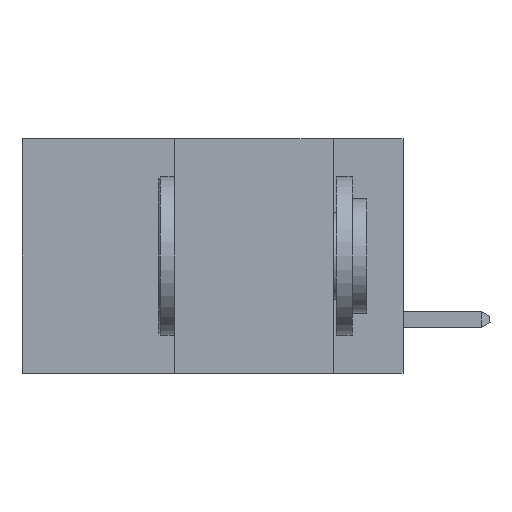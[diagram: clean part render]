
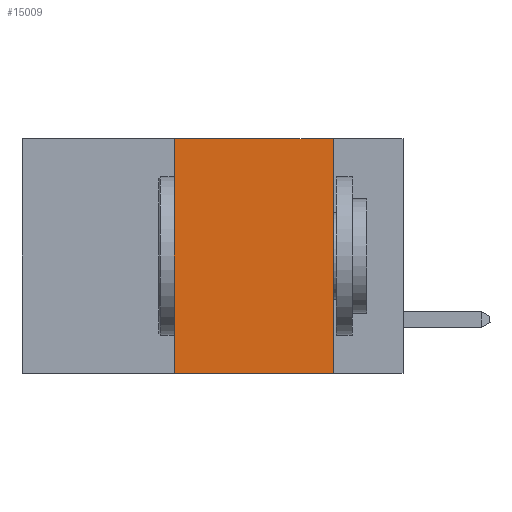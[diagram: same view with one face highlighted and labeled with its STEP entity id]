
A CAD part, left-side view. The second image highlights one B-rep face of the part: STEP entity #15009.
In plain terms, the highlighted planar face has unit normal (-1, 0, 0).
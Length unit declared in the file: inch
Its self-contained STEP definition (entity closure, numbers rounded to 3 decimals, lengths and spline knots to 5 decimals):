
#954 = EDGE_CURVE ( 'NONE', #8883, #10786, #8294, .T. ) ;
#1564 = ORIENTED_EDGE ( 'NONE', *, *, #954, .F. ) ;
#3146 = CARTESIAN_POINT ( 'NONE',  ( 0., 0.11, -0.37 ) ) ;
#3735 = DIRECTION ( 'NONE',  ( 0., -1., 0. ) ) ;
#4073 = VECTOR ( 'NONE', #7218, 39.37008 ) ;
#4391 = CARTESIAN_POINT ( 'NONE',  ( 0., 0.6, 0. ) ) ;
#4557 = ORIENTED_EDGE ( 'NONE', *, *, #16565, .T. ) ;
#4887 = CARTESIAN_POINT ( 'NONE',  ( 0., 0.36, -0.37 ) ) ;
#5022 = EDGE_LOOP ( 'NONE', ( #1564, #17696, #13849, #4557 ) ) ;
#5976 = FACE_OUTER_BOUND ( 'NONE', #5022, .T. ) ;
#6157 = DIRECTION ( 'NONE',  ( 0., 0., 1. ) ) ;
#6359 = VECTOR ( 'NONE', #3735, 39.37008 ) ;
#6648 = DIRECTION ( 'NONE',  ( 0., 0., -1. ) ) ;
#7033 = VECTOR ( 'NONE', #6157, 39.37008 ) ;
#7218 = DIRECTION ( 'NONE',  ( 0., -1., 0. ) ) ;
#7556 = EDGE_CURVE ( 'NONE', #12034, #14088, #10557, .T. ) ;
#8294 = LINE ( 'NONE', #17028, #17697 ) ;
#8883 = VERTEX_POINT ( 'NONE', #14789 ) ;
#10557 = LINE ( 'NONE', #13651, #7033 ) ;
#10786 = VERTEX_POINT ( 'NONE', #3146 ) ;
#11636 = CARTESIAN_POINT ( 'NONE',  ( 0., 0.36, 0. ) ) ;
#12034 = VERTEX_POINT ( 'NONE', #4887 ) ;
#13552 = PLANE ( 'NONE',  #14344 ) ;
#13640 = EDGE_CURVE ( 'NONE', #14088, #8883, #15729, .T. ) ;
#13651 = CARTESIAN_POINT ( 'NONE',  ( 0., 0.36, 0. ) ) ;
#13849 = ORIENTED_EDGE ( 'NONE', *, *, #7556, .F. ) ;
#14088 = VERTEX_POINT ( 'NONE', #11636 ) ;
#14344 = AXIS2_PLACEMENT_3D ( 'NONE', #17787, #16582, #6648 ) ;
#14789 = CARTESIAN_POINT ( 'NONE',  ( 0., 0.11, 0. ) ) ;
#15009 = ADVANCED_FACE ( 'NONE', ( #5976 ), #13552, .F. ) ;
#15729 = LINE ( 'NONE', #4391, #4073 ) ;
#15885 = DIRECTION ( 'NONE',  ( 0., 0., -1. ) ) ;
#16565 = EDGE_CURVE ( 'NONE', #12034, #10786, #17971, .T. ) ;
#16582 = DIRECTION ( 'NONE',  ( 1., 0., 0. ) ) ;
#17028 = CARTESIAN_POINT ( 'NONE',  ( 0., 0.11, 0. ) ) ;
#17696 = ORIENTED_EDGE ( 'NONE', *, *, #13640, .F. ) ;
#17697 = VECTOR ( 'NONE', #15885, 39.37008 ) ;
#17787 = CARTESIAN_POINT ( 'NONE',  ( 0., 0.6, 0. ) ) ;
#17842 = CARTESIAN_POINT ( 'NONE',  ( 0., 0.6, -0.37 ) ) ;
#17971 = LINE ( 'NONE', #17842, #6359 ) ;
